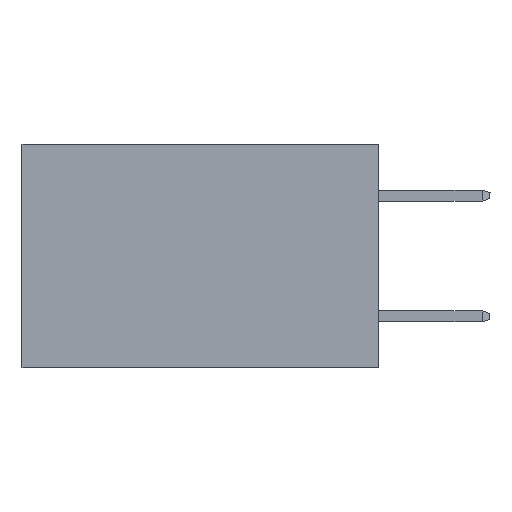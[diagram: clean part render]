
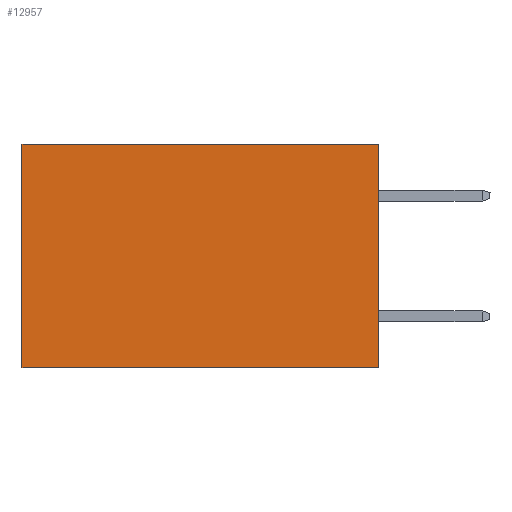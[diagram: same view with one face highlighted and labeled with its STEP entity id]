
A CAD part, left-side view. The second image highlights one B-rep face of the part: STEP entity #12957.
In plain terms, the highlighted planar face has unit normal (-1, 0, 0).
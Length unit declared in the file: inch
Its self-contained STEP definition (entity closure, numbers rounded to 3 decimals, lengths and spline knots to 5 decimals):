
#114 = AXIS2_PLACEMENT_3D ( 'NONE', #5305, #3251, #10492 ) ;
#128 = DIRECTION ( 'NONE',  ( 0., 0., -1. ) ) ;
#257 = VECTOR ( 'NONE', #1831, 39.37008 ) ;
#559 = ORIENTED_EDGE ( 'NONE', *, *, #1813, .T. ) ;
#1150 = CARTESIAN_POINT ( 'NONE',  ( 0.277, 0., -0.37 ) ) ;
#1216 = VERTEX_POINT ( 'NONE', #4989 ) ;
#1813 = EDGE_CURVE ( 'NONE', #7044, #10991, #2984, .T. ) ;
#1831 = DIRECTION ( 'NONE',  ( 0., 1., 0. ) ) ;
#2196 = LINE ( 'NONE', #3217, #12839 ) ;
#2221 = FACE_OUTER_BOUND ( 'NONE', #4436, .T. ) ;
#2434 = VECTOR ( 'NONE', #128, 39.37008 ) ;
#2898 = VECTOR ( 'NONE', #12175, 39.37008 ) ;
#2984 = LINE ( 'NONE', #12083, #257 ) ;
#3217 = CARTESIAN_POINT ( 'NONE',  ( 0.277, 0.59, -0.37 ) ) ;
#3251 = DIRECTION ( 'NONE',  ( 1., 0., 0. ) ) ;
#3272 = CARTESIAN_POINT ( 'NONE',  ( 0.277, 0., 0. ) ) ;
#3902 = EDGE_CURVE ( 'NONE', #7044, #10061, #7887, .T. ) ;
#4436 = EDGE_LOOP ( 'NONE', ( #11122, #7670, #5249, #559 ) ) ;
#4989 = CARTESIAN_POINT ( 'NONE',  ( 0.277, 0.59, -0.37 ) ) ;
#5249 = ORIENTED_EDGE ( 'NONE', *, *, #3902, .F. ) ;
#5305 = CARTESIAN_POINT ( 'NONE',  ( 0.277, 0., -0.37 ) ) ;
#5852 = EDGE_CURVE ( 'NONE', #10991, #1216, #2196, .T. ) ;
#6339 = DIRECTION ( 'NONE',  ( 0., 0., -1. ) ) ;
#6406 = CARTESIAN_POINT ( 'NONE',  ( 0.277, 0., -0.37 ) ) ;
#7044 = VERTEX_POINT ( 'NONE', #3272 ) ;
#7047 = CARTESIAN_POINT ( 'NONE',  ( 0.277, 0., -0.37 ) ) ;
#7670 = ORIENTED_EDGE ( 'NONE', *, *, #9597, .F. ) ;
#7887 = LINE ( 'NONE', #1150, #2434 ) ;
#7980 = CARTESIAN_POINT ( 'NONE',  ( 0.277, 0.59, 0. ) ) ;
#9454 = PLANE ( 'NONE',  #114 ) ;
#9597 = EDGE_CURVE ( 'NONE', #10061, #1216, #11138, .T. ) ;
#10061 = VERTEX_POINT ( 'NONE', #6406 ) ;
#10492 = DIRECTION ( 'NONE',  ( 0., 0., -1. ) ) ;
#10991 = VERTEX_POINT ( 'NONE', #7980 ) ;
#11122 = ORIENTED_EDGE ( 'NONE', *, *, #5852, .T. ) ;
#11138 = LINE ( 'NONE', #7047, #2898 ) ;
#12083 = CARTESIAN_POINT ( 'NONE',  ( 0.277, 0., 0. ) ) ;
#12175 = DIRECTION ( 'NONE',  ( 0., 1., 0. ) ) ;
#12839 = VECTOR ( 'NONE', #6339, 39.37008 ) ;
#12957 = ADVANCED_FACE ( 'NONE', ( #2221 ), #9454, .F. ) ;
